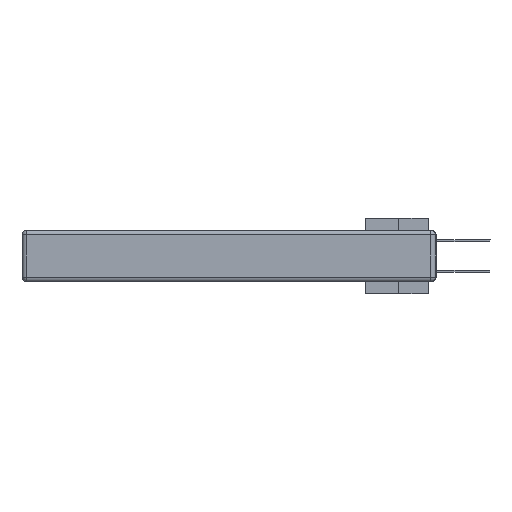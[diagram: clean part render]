
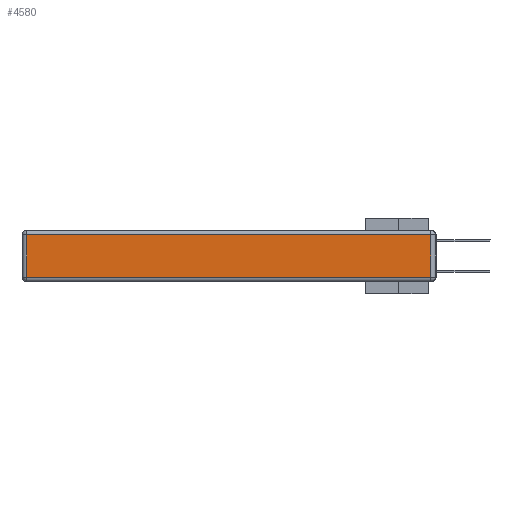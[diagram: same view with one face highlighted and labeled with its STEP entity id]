
A CAD part, left-side view. The second image highlights one B-rep face of the part: STEP entity #4580.
In plain terms, the highlighted planar face has unit normal (-1, 0, 0).
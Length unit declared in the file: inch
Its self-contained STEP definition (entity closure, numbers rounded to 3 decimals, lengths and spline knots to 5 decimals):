
#171 = VERTEX_POINT ( 'NONE', #24257 ) ;
#569 = ORIENTED_EDGE ( 'NONE', *, *, #22052, .T. ) ;
#985 = EDGE_CURVE ( 'NONE', #1504, #22915, #22984, .T. ) ;
#1247 = LINE ( 'NONE', #31096, #6958 ) ;
#1504 = VERTEX_POINT ( 'NONE', #17733 ) ;
#2551 = EDGE_CURVE ( 'NONE', #171, #1504, #19443, .T. ) ;
#3263 = CARTESIAN_POINT ( 'NONE',  ( 0., 0., -0.313 ) ) ;
#4580 = ADVANCED_FACE ( 'NONE', ( #20548 ), #31866, .T. ) ;
#4675 = CARTESIAN_POINT ( 'NONE',  ( 0., 2.72, -0.343 ) ) ;
#6958 = VECTOR ( 'NONE', #28058, 39.37008 ) ;
#7236 = CARTESIAN_POINT ( 'NONE',  ( 0., 0., -0.343 ) ) ;
#8828 = DIRECTION ( 'NONE',  ( 0., -1., 0. ) ) ;
#12408 = AXIS2_PLACEMENT_3D ( 'NONE', #7236, #15159, #23417 ) ;
#14585 = ORIENTED_EDGE ( 'NONE', *, *, #2551, .T. ) ;
#15159 = DIRECTION ( 'NONE',  ( -1., 0., 0. ) ) ;
#17733 = CARTESIAN_POINT ( 'NONE',  ( 0., 0.03, -0.313 ) ) ;
#18128 = VECTOR ( 'NONE', #35039, 39.37008 ) ;
#19443 = LINE ( 'NONE', #3263, #30507 ) ;
#19501 = EDGE_LOOP ( 'NONE', ( #14585, #31146, #33802, #569 ) ) ;
#20548 = FACE_OUTER_BOUND ( 'NONE', #19501, .T. ) ;
#21227 = VERTEX_POINT ( 'NONE', #26347 ) ;
#22052 = EDGE_CURVE ( 'NONE', #21227, #171, #32173, .T. ) ;
#22915 = VERTEX_POINT ( 'NONE', #25615 ) ;
#22984 = LINE ( 'NONE', #28219, #30441 ) ;
#23417 = DIRECTION ( 'NONE',  ( 0., 0., 1. ) ) ;
#24257 = CARTESIAN_POINT ( 'NONE',  ( 0., 2.72, -0.313 ) ) ;
#25615 = CARTESIAN_POINT ( 'NONE',  ( 0., 0.03, -0.03 ) ) ;
#26044 = DIRECTION ( 'NONE',  ( 0., 0., 1. ) ) ;
#26347 = CARTESIAN_POINT ( 'NONE',  ( 0., 2.72, -0.03 ) ) ;
#26817 = EDGE_CURVE ( 'NONE', #22915, #21227, #1247, .T. ) ;
#28058 = DIRECTION ( 'NONE',  ( 0., 1., 0. ) ) ;
#28219 = CARTESIAN_POINT ( 'NONE',  ( 0., 0.03, -0.343 ) ) ;
#30441 = VECTOR ( 'NONE', #26044, 39.37008 ) ;
#30507 = VECTOR ( 'NONE', #8828, 39.37008 ) ;
#31096 = CARTESIAN_POINT ( 'NONE',  ( 0., 2.75, -0.03 ) ) ;
#31146 = ORIENTED_EDGE ( 'NONE', *, *, #985, .T. ) ;
#31866 = PLANE ( 'NONE',  #12408 ) ;
#32173 = LINE ( 'NONE', #4675, #18128 ) ;
#33802 = ORIENTED_EDGE ( 'NONE', *, *, #26817, .T. ) ;
#35039 = DIRECTION ( 'NONE',  ( 0., 0., -1. ) ) ;
